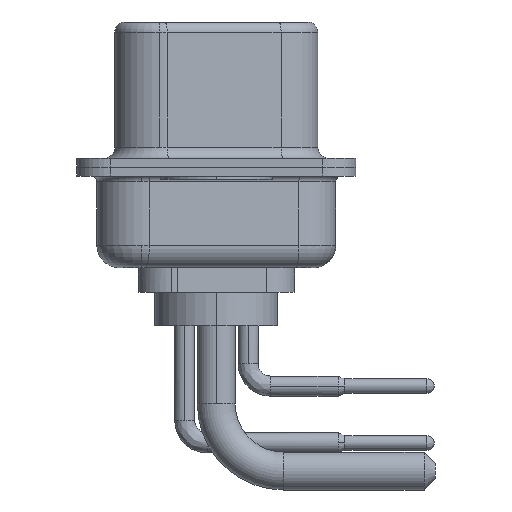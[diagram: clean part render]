
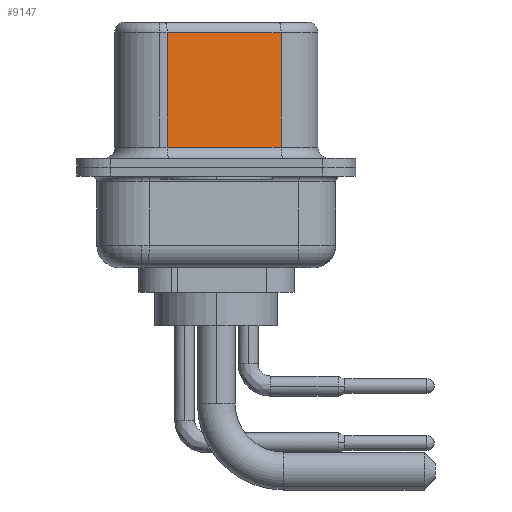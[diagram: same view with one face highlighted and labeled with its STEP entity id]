
A CAD part, left-side view. The second image highlights one B-rep face of the part: STEP entity #9147.
In plain terms, the highlighted planar face has unit normal (-0.985, -0.174, 0).
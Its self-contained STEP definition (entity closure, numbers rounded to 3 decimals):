
#135 = CARTESIAN_POINT ( 'NONE',  ( 4.58, -2.897, 6.02 ) ) ;
#1560 = LINE ( 'NONE', #135, #11440 ) ;
#1744 = VECTOR ( 'NONE', #19178, 1000. ) ;
#2600 = VERTEX_POINT ( 'NONE', #19934 ) ;
#2657 = EDGE_CURVE ( 'NONE', #8652, #2600, #16357, .T. ) ;
#2860 = EDGE_LOOP ( 'NONE', ( #4259, #20689, #7474, #20726 ) ) ;
#3603 = CARTESIAN_POINT ( 'NONE',  ( 3.68, 2.203, 6.52 ) ) ;
#3772 = AXIS2_PLACEMENT_3D ( 'NONE', #20515, #16694, #13570 ) ;
#4259 = ORIENTED_EDGE ( 'NONE', *, *, #11976, .F. ) ;
#5526 = CARTESIAN_POINT ( 'NONE',  ( 4.58, -2.897, 6.02 ) ) ;
#6263 = PLANE ( 'NONE',  #3772 ) ;
#7266 = CARTESIAN_POINT ( 'NONE',  ( 4.58, -2.897, 6.52 ) ) ;
#7474 = ORIENTED_EDGE ( 'NONE', *, *, #8825, .T. ) ;
#7502 = LINE ( 'NONE', #7266, #22050 ) ;
#8652 = VERTEX_POINT ( 'NONE', #21501 ) ;
#8825 = EDGE_CURVE ( 'NONE', #16796, #8652, #21103, .T. ) ;
#9074 = CARTESIAN_POINT ( 'NONE',  ( 3.68, 2.203, 6.02 ) ) ;
#9147 = ADVANCED_FACE ( 'NONE', ( #22146 ), #6263, .F. ) ;
#10476 = DIRECTION ( 'NONE',  ( -0.174, 0.985, 0. ) ) ;
#10858 = DIRECTION ( 'NONE',  ( 0., 0., -1. ) ) ;
#10901 = CARTESIAN_POINT ( 'NONE',  ( 4.58, -2.897, 0.9 ) ) ;
#11440 = VECTOR ( 'NONE', #10476, 1000. ) ;
#11901 = VERTEX_POINT ( 'NONE', #5526 ) ;
#11976 = EDGE_CURVE ( 'NONE', #11901, #2600, #7502, .T. ) ;
#12396 = DIRECTION ( 'NONE',  ( 0., 0., -1. ) ) ;
#12495 = VECTOR ( 'NONE', #12396, 1000. ) ;
#13570 = DIRECTION ( 'NONE',  ( -0.174, 0.985, 0. ) ) ;
#16357 = LINE ( 'NONE', #10901, #1744 ) ;
#16664 = EDGE_CURVE ( 'NONE', #11901, #16796, #1560, .T. ) ;
#16694 = DIRECTION ( 'NONE',  ( 0.985, 0.174, 0. ) ) ;
#16796 = VERTEX_POINT ( 'NONE', #9074 ) ;
#19178 = DIRECTION ( 'NONE',  ( 0.174, -0.985, 0. ) ) ;
#19934 = CARTESIAN_POINT ( 'NONE',  ( 4.58, -2.897, 0.9 ) ) ;
#20515 = CARTESIAN_POINT ( 'NONE',  ( 4.58, -2.897, 6.52 ) ) ;
#20689 = ORIENTED_EDGE ( 'NONE', *, *, #16664, .T. ) ;
#20726 = ORIENTED_EDGE ( 'NONE', *, *, #2657, .T. ) ;
#21103 = LINE ( 'NONE', #3603, #12495 ) ;
#21501 = CARTESIAN_POINT ( 'NONE',  ( 3.68, 2.203, 0.9 ) ) ;
#22050 = VECTOR ( 'NONE', #10858, 1000. ) ;
#22146 = FACE_OUTER_BOUND ( 'NONE', #2860, .T. ) ;
